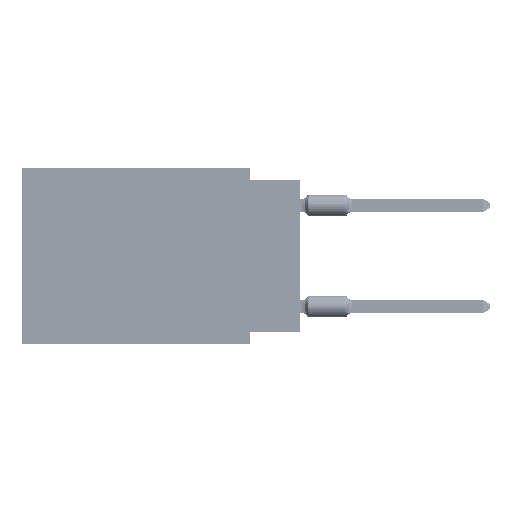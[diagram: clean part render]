
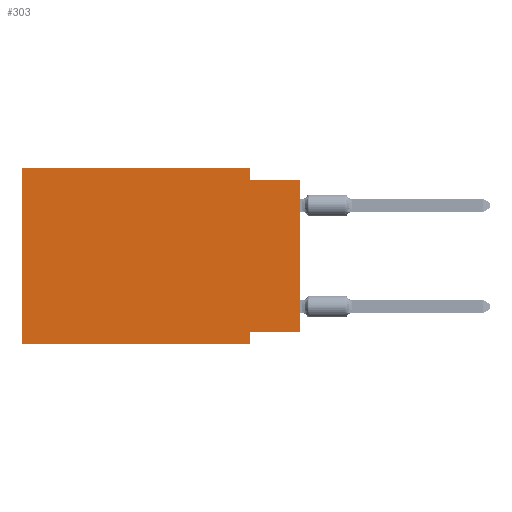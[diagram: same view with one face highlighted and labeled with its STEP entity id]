
A CAD part, left-side view. The second image highlights one B-rep face of the part: STEP entity #303.
In plain terms, the highlighted planar face has unit normal (-1, 0, 0).
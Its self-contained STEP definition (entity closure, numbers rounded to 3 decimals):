
#247 = VECTOR ( 'NONE', #22258, 1000. ) ;
#303 = ADVANCED_FACE ( 'NONE', ( #12167 ), #13952, .F. ) ;
#5125 = EDGE_CURVE ( 'NONE', #63978, #74409, #35569, .T. ) ;
#5904 = VECTOR ( 'NONE', #43100, 1000. ) ;
#7955 = EDGE_CURVE ( 'NONE', #74409, #8175, #8058, .T. ) ;
#8058 = LINE ( 'NONE', #73690, #45662 ) ;
#8175 = VERTEX_POINT ( 'NONE', #28207 ) ;
#10926 = CARTESIAN_POINT ( 'NONE',  ( 0., 0., -8.255 ) ) ;
#11367 = DIRECTION ( 'NONE',  ( 0., 0., 1. ) ) ;
#11753 = DIRECTION ( 'NONE',  ( 0., -1., 0. ) ) ;
#12167 = FACE_OUTER_BOUND ( 'NONE', #51510, .T. ) ;
#13952 = PLANE ( 'NONE',  #72307 ) ;
#14830 = CARTESIAN_POINT ( 'NONE',  ( 0., 2.54, 0. ) ) ;
#17386 = CARTESIAN_POINT ( 'NONE',  ( 0., 13.97, 0. ) ) ;
#18374 = ORIENTED_EDGE ( 'NONE', *, *, #5125, .F. ) ;
#18584 = VERTEX_POINT ( 'NONE', #17386 ) ;
#18609 = LINE ( 'NONE', #77516, #23262 ) ;
#21864 = LINE ( 'NONE', #34900, #5904 ) ;
#22125 = ORIENTED_EDGE ( 'NONE', *, *, #53378, .T. ) ;
#22258 = DIRECTION ( 'NONE',  ( 0., 0., -1. ) ) ;
#23262 = VECTOR ( 'NONE', #11367, 1000. ) ;
#24132 = EDGE_CURVE ( 'NONE', #83245, #65978, #95158, .T. ) ;
#26811 = EDGE_CURVE ( 'NONE', #18584, #63978, #94770, .T. ) ;
#27178 = VECTOR ( 'NONE', #89200, 1000. ) ;
#28207 = CARTESIAN_POINT ( 'NONE',  ( 0., 0., -0.635 ) ) ;
#29006 = CARTESIAN_POINT ( 'NONE',  ( 0., 2.54, -8.89 ) ) ;
#30032 = CARTESIAN_POINT ( 'NONE',  ( 0., 2.54, -0.635 ) ) ;
#30814 = EDGE_CURVE ( 'NONE', #43196, #8175, #90146, .T. ) ;
#34610 = CARTESIAN_POINT ( 'NONE',  ( 0., 2.54, -8.255 ) ) ;
#34900 = CARTESIAN_POINT ( 'NONE',  ( 0., 0., -8.255 ) ) ;
#35060 = EDGE_CURVE ( 'NONE', #43196, #83245, #21864, .T. ) ;
#35569 = LINE ( 'NONE', #14830, #82273 ) ;
#38301 = ORIENTED_EDGE ( 'NONE', *, *, #26811, .F. ) ;
#38520 = DIRECTION ( 'NONE',  ( 0., 0., -1. ) ) ;
#41185 = CARTESIAN_POINT ( 'NONE',  ( 0., 13.97, 0. ) ) ;
#43100 = DIRECTION ( 'NONE',  ( 0., 1., 0. ) ) ;
#43196 = VERTEX_POINT ( 'NONE', #10926 ) ;
#43379 = CARTESIAN_POINT ( 'NONE',  ( 0., 13.97, 0. ) ) ;
#45253 = CARTESIAN_POINT ( 'NONE',  ( 0., 0., 0. ) ) ;
#45662 = VECTOR ( 'NONE', #46120, 1000. ) ;
#46120 = DIRECTION ( 'NONE',  ( 0., -1., 0. ) ) ;
#47467 = ORIENTED_EDGE ( 'NONE', *, *, #7955, .F. ) ;
#47816 = CARTESIAN_POINT ( 'NONE',  ( 0., 2.54, 0. ) ) ;
#48780 = ORIENTED_EDGE ( 'NONE', *, *, #30814, .T. ) ;
#50140 = VERTEX_POINT ( 'NONE', #75285 ) ;
#50555 = DIRECTION ( 'NONE',  ( 0., 0., -1. ) ) ;
#51510 = EDGE_LOOP ( 'NONE', ( #48780, #47467, #18374, #38301, #59407, #22125, #68056, #90173 ) ) ;
#53378 = EDGE_CURVE ( 'NONE', #50140, #65978, #93475, .T. ) ;
#55902 = VECTOR ( 'NONE', #11753, 1000. ) ;
#59315 = DIRECTION ( 'NONE',  ( 1., 0., 0. ) ) ;
#59407 = ORIENTED_EDGE ( 'NONE', *, *, #70406, .F. ) ;
#63978 = VERTEX_POINT ( 'NONE', #47816 ) ;
#65978 = VERTEX_POINT ( 'NONE', #91086 ) ;
#68056 = ORIENTED_EDGE ( 'NONE', *, *, #24132, .F. ) ;
#69725 = VECTOR ( 'NONE', #71742, 1000. ) ;
#70406 = EDGE_CURVE ( 'NONE', #50140, #18584, #18609, .T. ) ;
#71742 = DIRECTION ( 'NONE',  ( 0., -1., 0. ) ) ;
#72307 = AXIS2_PLACEMENT_3D ( 'NONE', #43379, #59315, #38520 ) ;
#73690 = CARTESIAN_POINT ( 'NONE',  ( 0., 0., -0.635 ) ) ;
#74409 = VERTEX_POINT ( 'NONE', #30032 ) ;
#75285 = CARTESIAN_POINT ( 'NONE',  ( 0., 13.97, -8.89 ) ) ;
#77516 = CARTESIAN_POINT ( 'NONE',  ( 0., 13.97, 0. ) ) ;
#82273 = VECTOR ( 'NONE', #50555, 1000. ) ;
#83245 = VERTEX_POINT ( 'NONE', #34610 ) ;
#87185 = CARTESIAN_POINT ( 'NONE',  ( 0., 13.97, -8.89 ) ) ;
#89200 = DIRECTION ( 'NONE',  ( 0., 0., 1. ) ) ;
#90146 = LINE ( 'NONE', #45253, #27178 ) ;
#90173 = ORIENTED_EDGE ( 'NONE', *, *, #35060, .F. ) ;
#91086 = CARTESIAN_POINT ( 'NONE',  ( 0., 2.54, -8.89 ) ) ;
#93475 = LINE ( 'NONE', #87185, #69725 ) ;
#94770 = LINE ( 'NONE', #41185, #55902 ) ;
#95158 = LINE ( 'NONE', #29006, #247 ) ;
